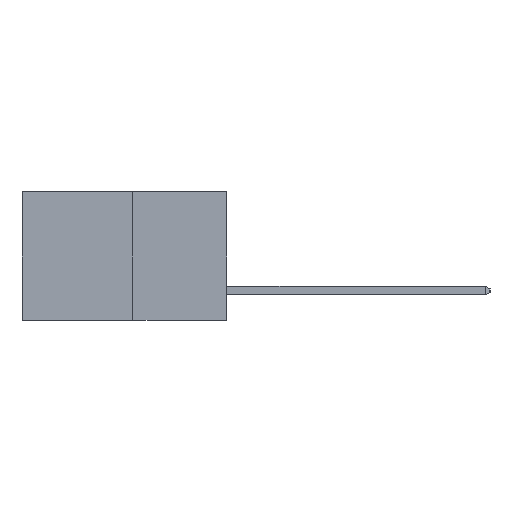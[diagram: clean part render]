
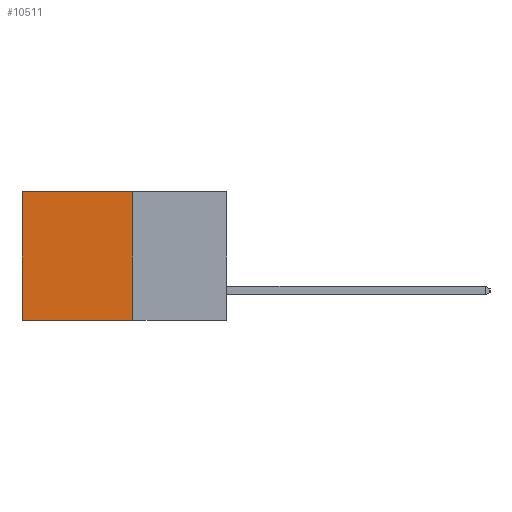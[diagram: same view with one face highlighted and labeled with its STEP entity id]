
A CAD part, left-side view. The second image highlights one B-rep face of the part: STEP entity #10511.
In plain terms, the highlighted planar face has unit normal (-1, 0, 0).
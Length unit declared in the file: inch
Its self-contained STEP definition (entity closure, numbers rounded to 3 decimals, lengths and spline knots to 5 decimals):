
#770 = EDGE_CURVE ( 'NONE', #5336, #11752, #8460, .T. ) ;
#884 = DIRECTION ( 'NONE',  ( 0., 0., -1. ) ) ;
#968 = ORIENTED_EDGE ( 'NONE', *, *, #770, .F. ) ;
#1454 = EDGE_CURVE ( 'NONE', #1749, #8525, #5966, .T. ) ;
#1749 = VERTEX_POINT ( 'NONE', #6121 ) ;
#2020 = CARTESIAN_POINT ( 'NONE',  ( 0.277, 0.59, -0.37 ) ) ;
#2183 = CARTESIAN_POINT ( 'NONE',  ( 0.277, 0.27, 0. ) ) ;
#2856 = CARTESIAN_POINT ( 'NONE',  ( 0.277, 0.27, -0.37 ) ) ;
#2869 = EDGE_CURVE ( 'NONE', #5336, #1749, #10091, .T. ) ;
#3096 = VECTOR ( 'NONE', #9614, 39.37008 ) ;
#3279 = EDGE_LOOP ( 'NONE', ( #12046, #4838, #968, #7693 ) ) ;
#3350 = VECTOR ( 'NONE', #884, 39.37008 ) ;
#3492 = DIRECTION ( 'NONE',  ( 1., 0., 0. ) ) ;
#3930 = FACE_OUTER_BOUND ( 'NONE', #3279, .T. ) ;
#4127 = CARTESIAN_POINT ( 'NONE',  ( 0.277, 0.59, -0.37 ) ) ;
#4838 = ORIENTED_EDGE ( 'NONE', *, *, #6388, .F. ) ;
#4846 = CARTESIAN_POINT ( 'NONE',  ( 0.277, 0.27, -0.37 ) ) ;
#5336 = VERTEX_POINT ( 'NONE', #6530 ) ;
#5966 = LINE ( 'NONE', #4127, #10696 ) ;
#6121 = CARTESIAN_POINT ( 'NONE',  ( 0.277, 0.59, 0. ) ) ;
#6388 = EDGE_CURVE ( 'NONE', #11752, #8525, #10735, .T. ) ;
#6530 = CARTESIAN_POINT ( 'NONE',  ( 0.277, 0.27, 0. ) ) ;
#7693 = ORIENTED_EDGE ( 'NONE', *, *, #2869, .T. ) ;
#8271 = PLANE ( 'NONE',  #10067 ) ;
#8411 = CARTESIAN_POINT ( 'NONE',  ( 0.277, 0.27, -0.37 ) ) ;
#8460 = LINE ( 'NONE', #4846, #3350 ) ;
#8525 = VERTEX_POINT ( 'NONE', #2020 ) ;
#9213 = CARTESIAN_POINT ( 'NONE',  ( 0.277, 0.27, -0.37 ) ) ;
#9361 = DIRECTION ( 'NONE',  ( 0., 0., -1. ) ) ;
#9614 = DIRECTION ( 'NONE',  ( 0., 1., 0. ) ) ;
#10067 = AXIS2_PLACEMENT_3D ( 'NONE', #9213, #3492, #10178 ) ;
#10091 = LINE ( 'NONE', #2183, #12192 ) ;
#10178 = DIRECTION ( 'NONE',  ( 0., 0., -1. ) ) ;
#10471 = DIRECTION ( 'NONE',  ( 0., 1., 0. ) ) ;
#10511 = ADVANCED_FACE ( 'NONE', ( #3930 ), #8271, .F. ) ;
#10696 = VECTOR ( 'NONE', #9361, 39.37008 ) ;
#10735 = LINE ( 'NONE', #2856, #3096 ) ;
#11752 = VERTEX_POINT ( 'NONE', #8411 ) ;
#12046 = ORIENTED_EDGE ( 'NONE', *, *, #1454, .T. ) ;
#12192 = VECTOR ( 'NONE', #10471, 39.37008 ) ;
